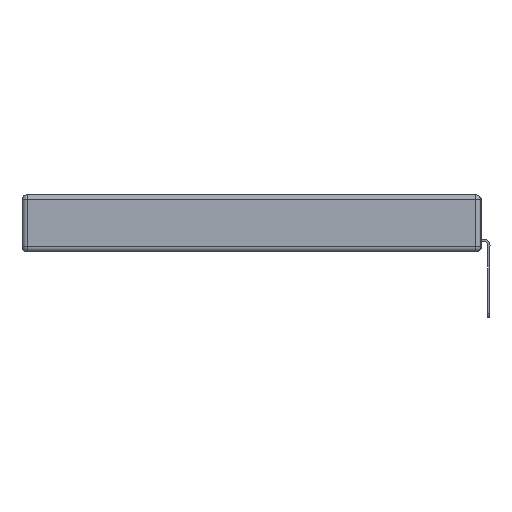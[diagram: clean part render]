
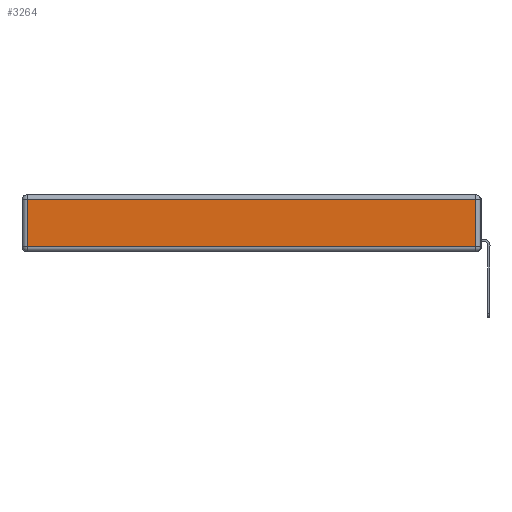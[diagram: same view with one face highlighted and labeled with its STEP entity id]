
A CAD part, left-side view. The second image highlights one B-rep face of the part: STEP entity #3264.
In plain terms, the highlighted planar face has unit normal (-1, 0, 0).
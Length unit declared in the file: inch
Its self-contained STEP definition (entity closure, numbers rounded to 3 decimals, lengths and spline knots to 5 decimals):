
#992 = ORIENTED_EDGE ( 'NONE', *, *, #20902, .T. ) ;
#2200 = CARTESIAN_POINT ( 'NONE',  ( 0., 0.03, -0.03 ) ) ;
#3081 = CARTESIAN_POINT ( 'NONE',  ( 0., 2.75, -0.03 ) ) ;
#3264 = ADVANCED_FACE ( 'NONE', ( #7370 ), #23099, .T. ) ;
#3777 = LINE ( 'NONE', #6221, #10755 ) ;
#3941 = CARTESIAN_POINT ( 'NONE',  ( 0., 2.72, -0.313 ) ) ;
#5009 = CARTESIAN_POINT ( 'NONE',  ( 0., 2.72, -0.03 ) ) ;
#6221 = CARTESIAN_POINT ( 'NONE',  ( 0., 0.03, -0.343 ) ) ;
#6315 = ORIENTED_EDGE ( 'NONE', *, *, #25991, .T. ) ;
#6706 = ORIENTED_EDGE ( 'NONE', *, *, #14105, .T. ) ;
#6823 = CARTESIAN_POINT ( 'NONE',  ( 0., 0., -0.343 ) ) ;
#7370 = FACE_OUTER_BOUND ( 'NONE', #9141, .T. ) ;
#7708 = VECTOR ( 'NONE', #13444, 39.37008 ) ;
#8858 = DIRECTION ( 'NONE',  ( -1., 0., 0. ) ) ;
#9141 = EDGE_LOOP ( 'NONE', ( #6706, #6315, #20615, #992 ) ) ;
#9466 = DIRECTION ( 'NONE',  ( 0., 0., -1. ) ) ;
#9695 = VERTEX_POINT ( 'NONE', #15853 ) ;
#10031 = EDGE_CURVE ( 'NONE', #17111, #25150, #11053, .T. ) ;
#10135 = LINE ( 'NONE', #11141, #18384 ) ;
#10230 = LINE ( 'NONE', #21724, #7708 ) ;
#10755 = VECTOR ( 'NONE', #12223, 39.37008 ) ;
#10895 = DIRECTION ( 'NONE',  ( 0., 0., 1. ) ) ;
#11053 = LINE ( 'NONE', #3081, #13587 ) ;
#11141 = CARTESIAN_POINT ( 'NONE',  ( 0., 2.72, -0.343 ) ) ;
#12223 = DIRECTION ( 'NONE',  ( 0., 0., 1. ) ) ;
#13084 = VERTEX_POINT ( 'NONE', #3941 ) ;
#13444 = DIRECTION ( 'NONE',  ( 0., -1., 0. ) ) ;
#13587 = VECTOR ( 'NONE', #23279, 39.37008 ) ;
#14105 = EDGE_CURVE ( 'NONE', #13084, #9695, #10230, .T. ) ;
#15853 = CARTESIAN_POINT ( 'NONE',  ( 0., 0.03, -0.313 ) ) ;
#17111 = VERTEX_POINT ( 'NONE', #2200 ) ;
#18384 = VECTOR ( 'NONE', #9466, 39.37008 ) ;
#20615 = ORIENTED_EDGE ( 'NONE', *, *, #10031, .T. ) ;
#20902 = EDGE_CURVE ( 'NONE', #25150, #13084, #10135, .T. ) ;
#21724 = CARTESIAN_POINT ( 'NONE',  ( 0., 0., -0.313 ) ) ;
#23099 = PLANE ( 'NONE',  #25354 ) ;
#23279 = DIRECTION ( 'NONE',  ( 0., 1., 0. ) ) ;
#25150 = VERTEX_POINT ( 'NONE', #5009 ) ;
#25354 = AXIS2_PLACEMENT_3D ( 'NONE', #6823, #8858, #10895 ) ;
#25991 = EDGE_CURVE ( 'NONE', #9695, #17111, #3777, .T. ) ;
